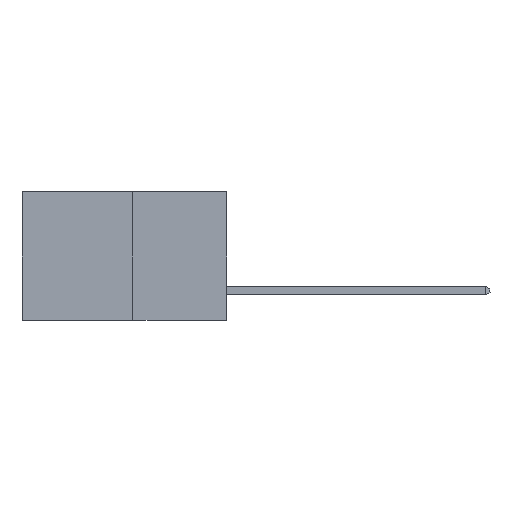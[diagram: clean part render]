
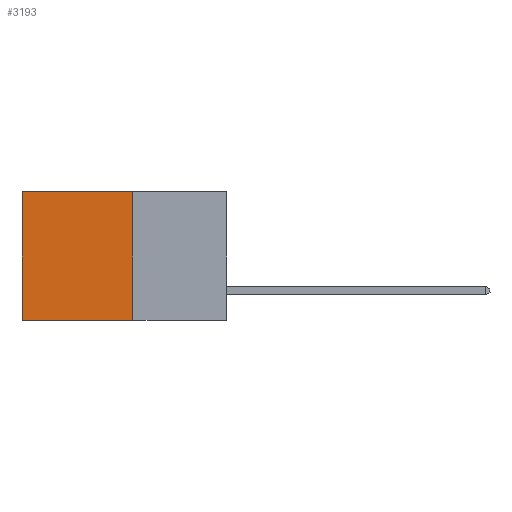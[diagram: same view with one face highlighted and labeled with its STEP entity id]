
A CAD part, left-side view. The second image highlights one B-rep face of the part: STEP entity #3193.
In plain terms, the highlighted planar face has unit normal (-1, 0, 0).
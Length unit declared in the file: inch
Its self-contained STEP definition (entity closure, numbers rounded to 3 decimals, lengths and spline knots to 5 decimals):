
#491 = DIRECTION ( 'NONE',  ( 0., 0., -1. ) ) ;
#1057 = EDGE_CURVE ( 'NONE', #12715, #6787, #11701, .T. ) ;
#1136 = ORIENTED_EDGE ( 'NONE', *, *, #11527, .F. ) ;
#1589 = ORIENTED_EDGE ( 'NONE', *, *, #1057, .T. ) ;
#1980 = DIRECTION ( 'NONE',  ( 0., 0., -1. ) ) ;
#2976 = CARTESIAN_POINT ( 'NONE',  ( 0.277, 0.27, -0.37 ) ) ;
#3193 = ADVANCED_FACE ( 'NONE', ( #3223 ), #5196, .F. ) ;
#3223 = FACE_OUTER_BOUND ( 'NONE', #9422, .T. ) ;
#4284 = VECTOR ( 'NONE', #491, 39.37008 ) ;
#4581 = CARTESIAN_POINT ( 'NONE',  ( 0.277, 0.59, 0. ) ) ;
#4680 = ORIENTED_EDGE ( 'NONE', *, *, #9510, .T. ) ;
#5061 = EDGE_CURVE ( 'NONE', #12715, #7056, #6883, .T. ) ;
#5196 = PLANE ( 'NONE',  #5846 ) ;
#5846 = AXIS2_PLACEMENT_3D ( 'NONE', #8094, #6166, #13148 ) ;
#5848 = CARTESIAN_POINT ( 'NONE',  ( 0.277, 0.27, 0. ) ) ;
#6104 = VECTOR ( 'NONE', #1980, 39.37008 ) ;
#6166 = DIRECTION ( 'NONE',  ( 1., 0., 0. ) ) ;
#6260 = DIRECTION ( 'NONE',  ( 0., 1., 0. ) ) ;
#6787 = VERTEX_POINT ( 'NONE', #4581 ) ;
#6883 = LINE ( 'NONE', #10560, #4284 ) ;
#7056 = VERTEX_POINT ( 'NONE', #2976 ) ;
#7114 = CARTESIAN_POINT ( 'NONE',  ( 0.277, 0.59, -0.37 ) ) ;
#7907 = DIRECTION ( 'NONE',  ( 0., 1., 0. ) ) ;
#7975 = CARTESIAN_POINT ( 'NONE',  ( 0.277, 0.59, -0.37 ) ) ;
#8044 = LINE ( 'NONE', #10197, #10329 ) ;
#8094 = CARTESIAN_POINT ( 'NONE',  ( 0.277, 0.27, -0.37 ) ) ;
#8928 = VERTEX_POINT ( 'NONE', #7114 ) ;
#9018 = VECTOR ( 'NONE', #7907, 39.37008 ) ;
#9422 = EDGE_LOOP ( 'NONE', ( #4680, #1136, #9686, #1589 ) ) ;
#9510 = EDGE_CURVE ( 'NONE', #6787, #8928, #11810, .T. ) ;
#9686 = ORIENTED_EDGE ( 'NONE', *, *, #5061, .F. ) ;
#10197 = CARTESIAN_POINT ( 'NONE',  ( 0.277, 0.27, -0.37 ) ) ;
#10329 = VECTOR ( 'NONE', #6260, 39.37008 ) ;
#10560 = CARTESIAN_POINT ( 'NONE',  ( 0.277, 0.27, -0.37 ) ) ;
#10747 = CARTESIAN_POINT ( 'NONE',  ( 0.277, 0.27, 0. ) ) ;
#11527 = EDGE_CURVE ( 'NONE', #7056, #8928, #8044, .T. ) ;
#11701 = LINE ( 'NONE', #10747, #9018 ) ;
#11810 = LINE ( 'NONE', #7975, #6104 ) ;
#12715 = VERTEX_POINT ( 'NONE', #5848 ) ;
#13148 = DIRECTION ( 'NONE',  ( 0., 0., -1. ) ) ;
